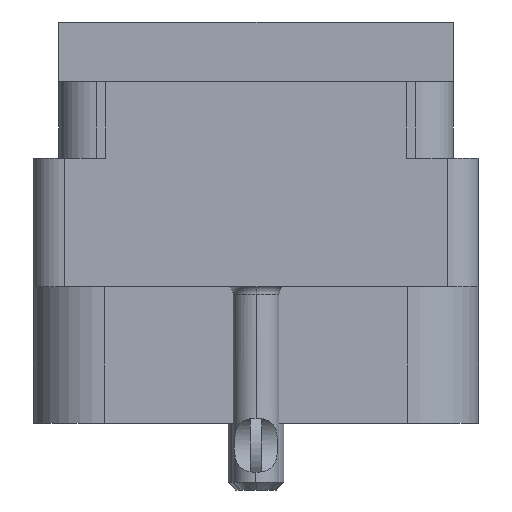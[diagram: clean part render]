
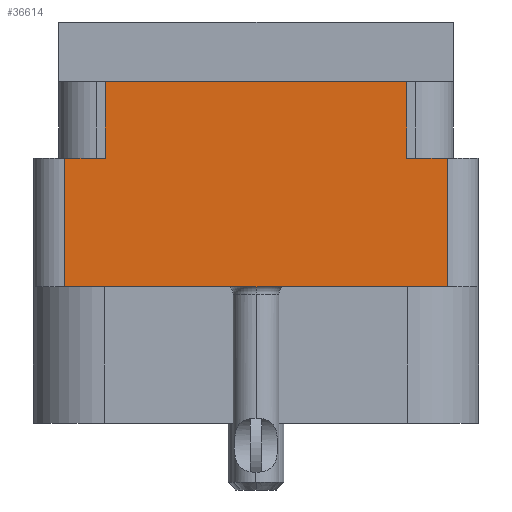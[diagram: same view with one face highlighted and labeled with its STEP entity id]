
A CAD part, left-side view. The second image highlights one B-rep face of the part: STEP entity #36614.
In plain terms, the highlighted planar face has unit normal (-1, 0, 0).
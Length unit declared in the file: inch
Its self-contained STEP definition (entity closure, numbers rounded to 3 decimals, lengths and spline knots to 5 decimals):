
#1329 = DIRECTION ( 'NONE',  ( 0., -1., 0. ) ) ;
#2899 = ORIENTED_EDGE ( 'NONE', *, *, #41179, .F. ) ;
#3277 = LINE ( 'NONE', #34084, #5925 ) ;
#3683 = CARTESIAN_POINT ( 'NONE',  ( -1., -0.438, -0.789 ) ) ;
#5263 = LINE ( 'NONE', #19790, #37923 ) ;
#5925 = VECTOR ( 'NONE', #10692, 39.37008 ) ;
#6243 = ORIENTED_EDGE ( 'NONE', *, *, #18907, .F. ) ;
#6468 = DIRECTION ( 'NONE',  ( 0., 0., 1. ) ) ;
#7777 = EDGE_LOOP ( 'NONE', ( #26271, #36751, #9144, #38121, #6243, #11597, #2899, #22261 ) ) ;
#9144 = ORIENTED_EDGE ( 'NONE', *, *, #19713, .T. ) ;
#10353 = VERTEX_POINT ( 'NONE', #21272 ) ;
#10692 = DIRECTION ( 'NONE',  ( 0., -1., 0. ) ) ;
#10975 = LINE ( 'NONE', #23142, #14566 ) ;
#11316 = CARTESIAN_POINT ( 'NONE',  ( -1., 0., -0.268 ) ) ;
#11597 = ORIENTED_EDGE ( 'NONE', *, *, #31499, .T. ) ;
#12530 = VECTOR ( 'NONE', #14760, 39.37008 ) ;
#13640 = DIRECTION ( 'NONE',  ( -1., 0., 0. ) ) ;
#13821 = DIRECTION ( 'NONE',  ( 0., 0., -1. ) ) ;
#14096 = VERTEX_POINT ( 'NONE', #40650 ) ;
#14173 = LINE ( 'NONE', #37113, #25142 ) ;
#14467 = EDGE_CURVE ( 'NONE', #29578, #14096, #35329, .T. ) ;
#14566 = VECTOR ( 'NONE', #19919, 39.37008 ) ;
#14760 = DIRECTION ( 'NONE',  ( 0., -1., 0. ) ) ;
#15940 = VERTEX_POINT ( 'NONE', #19754 ) ;
#16464 = CARTESIAN_POINT ( 'NONE',  ( -1., 0.296, -0.268 ) ) ;
#16927 = VERTEX_POINT ( 'NONE', #17749 ) ;
#17749 = CARTESIAN_POINT ( 'NONE',  ( -1., 0.376, -0.52 ) ) ;
#17931 = VECTOR ( 'NONE', #13821, 39.37008 ) ;
#18907 = EDGE_CURVE ( 'NONE', #33856, #15940, #3277, .T. ) ;
#19302 = LINE ( 'NONE', #30513, #12530 ) ;
#19713 = EDGE_CURVE ( 'NONE', #16927, #10353, #19302, .T. ) ;
#19754 = CARTESIAN_POINT ( 'NONE',  ( -1., -0.376, -0.268 ) ) ;
#19790 = CARTESIAN_POINT ( 'NONE',  ( -1., -0.376, -0.789 ) ) ;
#19919 = DIRECTION ( 'NONE',  ( 0., 0., 1. ) ) ;
#20074 = PLANE ( 'NONE',  #22433 ) ;
#21272 = CARTESIAN_POINT ( 'NONE',  ( -1., -0.376, -0.52 ) ) ;
#22261 = ORIENTED_EDGE ( 'NONE', *, *, #14467, .F. ) ;
#22433 = AXIS2_PLACEMENT_3D ( 'NONE', #3683, #13640, #6468 ) ;
#22846 = VECTOR ( 'NONE', #33718, 39.37008 ) ;
#23142 = CARTESIAN_POINT ( 'NONE',  ( -1., -0.296, -0.268 ) ) ;
#25142 = VECTOR ( 'NONE', #33758, 39.37008 ) ;
#26022 = VECTOR ( 'NONE', #1329, 39.37008 ) ;
#26271 = ORIENTED_EDGE ( 'NONE', *, *, #26937, .F. ) ;
#26795 = LINE ( 'NONE', #40303, #17931 ) ;
#26937 = EDGE_CURVE ( 'NONE', #34857, #29578, #27066, .T. ) ;
#27066 = LINE ( 'NONE', #11316, #26022 ) ;
#27791 = EDGE_CURVE ( 'NONE', #10353, #15940, #5263, .T. ) ;
#29578 = VERTEX_POINT ( 'NONE', #16464 ) ;
#30513 = CARTESIAN_POINT ( 'NONE',  ( -1., 0., -0.52 ) ) ;
#31499 = EDGE_CURVE ( 'NONE', #33856, #41468, #10975, .T. ) ;
#31979 = FACE_OUTER_BOUND ( 'NONE', #7777, .T. ) ;
#32017 = CARTESIAN_POINT ( 'NONE',  ( -1., 0.376, -0.268 ) ) ;
#32236 = CARTESIAN_POINT ( 'NONE',  ( -1., -0.296, -0.268 ) ) ;
#33718 = DIRECTION ( 'NONE',  ( 0., 0., 1. ) ) ;
#33758 = DIRECTION ( 'NONE',  ( 0., -1., 0. ) ) ;
#33856 = VERTEX_POINT ( 'NONE', #32236 ) ;
#34084 = CARTESIAN_POINT ( 'NONE',  ( -1., 0., -0.268 ) ) ;
#34857 = VERTEX_POINT ( 'NONE', #32017 ) ;
#35063 = CARTESIAN_POINT ( 'NONE',  ( -1., -0.296, -0.117 ) ) ;
#35329 = LINE ( 'NONE', #40542, #22846 ) ;
#36614 = ADVANCED_FACE ( 'NONE', ( #31979 ), #20074, .T. ) ;
#36751 = ORIENTED_EDGE ( 'NONE', *, *, #39280, .T. ) ;
#37113 = CARTESIAN_POINT ( 'NONE',  ( -1., 0.438, -0.117 ) ) ;
#37923 = VECTOR ( 'NONE', #39854, 39.37008 ) ;
#38121 = ORIENTED_EDGE ( 'NONE', *, *, #27791, .T. ) ;
#39280 = EDGE_CURVE ( 'NONE', #34857, #16927, #26795, .T. ) ;
#39854 = DIRECTION ( 'NONE',  ( 0., 0., 1. ) ) ;
#40303 = CARTESIAN_POINT ( 'NONE',  ( -1., 0.376, -0.789 ) ) ;
#40542 = CARTESIAN_POINT ( 'NONE',  ( -1., 0.296, -0.268 ) ) ;
#40650 = CARTESIAN_POINT ( 'NONE',  ( -1., 0.296, -0.117 ) ) ;
#41179 = EDGE_CURVE ( 'NONE', #14096, #41468, #14173, .T. ) ;
#41468 = VERTEX_POINT ( 'NONE', #35063 ) ;
